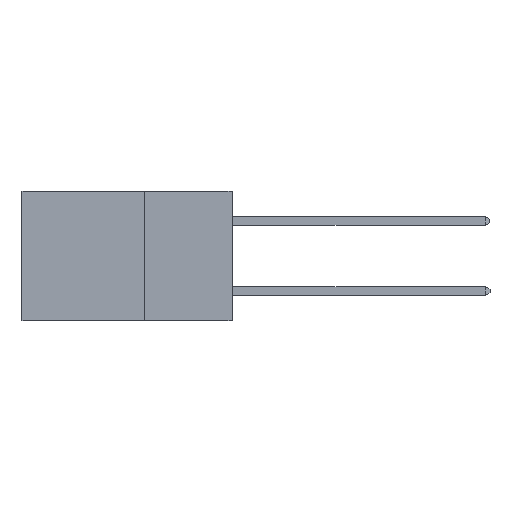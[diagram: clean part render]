
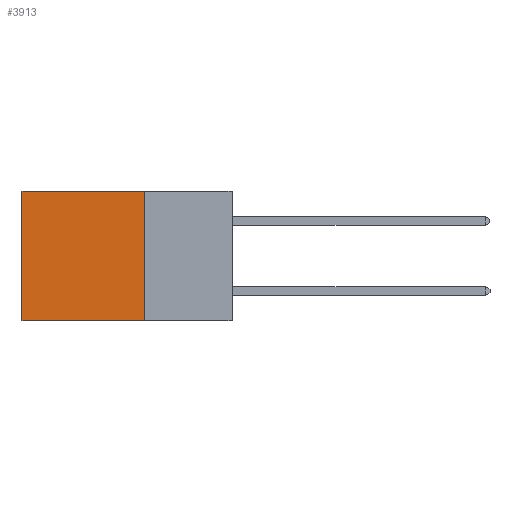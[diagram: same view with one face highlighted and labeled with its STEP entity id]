
A CAD part, left-side view. The second image highlights one B-rep face of the part: STEP entity #3913.
In plain terms, the highlighted planar face has unit normal (-1, 0, 0).
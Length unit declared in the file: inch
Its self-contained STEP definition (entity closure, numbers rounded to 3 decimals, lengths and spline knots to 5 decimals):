
#161 = VERTEX_POINT ( 'NONE', #17658 ) ;
#2437 = EDGE_CURVE ( 'NONE', #161, #13898, #17743, .T. ) ;
#3913 = ADVANCED_FACE ( 'NONE', ( #23017 ), #18521, .F. ) ;
#4895 = AXIS2_PLACEMENT_3D ( 'NONE', #5978, #7819, #20319 ) ;
#4899 = DIRECTION ( 'NONE',  ( 0., 0., -1. ) ) ;
#5817 = CARTESIAN_POINT ( 'NONE',  ( 0.2875, 0.25, -0.37 ) ) ;
#5978 = CARTESIAN_POINT ( 'NONE',  ( 0.2875, 0.25, 0. ) ) ;
#6065 = EDGE_LOOP ( 'NONE', ( #21045, #9711, #15027, #20027 ) ) ;
#6072 = EDGE_CURVE ( 'NONE', #22263, #13898, #16284, .T. ) ;
#6254 = CARTESIAN_POINT ( 'NONE',  ( 0.2875, 0.25, 0. ) ) ;
#6277 = EDGE_CURVE ( 'NONE', #7424, #22263, #7571, .T. ) ;
#6336 = DIRECTION ( 'NONE',  ( 0., 0., -1. ) ) ;
#7301 = CARTESIAN_POINT ( 'NONE',  ( 0.2875, 0.25, 0. ) ) ;
#7424 = VERTEX_POINT ( 'NONE', #19966 ) ;
#7571 = LINE ( 'NONE', #7301, #21841 ) ;
#7819 = DIRECTION ( 'NONE',  ( 1., 0., 0. ) ) ;
#8804 = VECTOR ( 'NONE', #11307, 39.37008 ) ;
#9711 = ORIENTED_EDGE ( 'NONE', *, *, #2437, .F. ) ;
#10094 = EDGE_CURVE ( 'NONE', #7424, #161, #15143, .T. ) ;
#11307 = DIRECTION ( 'NONE',  ( 0., 1., 0. ) ) ;
#13898 = VERTEX_POINT ( 'NONE', #19882 ) ;
#14574 = VECTOR ( 'NONE', #6336, 39.37008 ) ;
#15027 = ORIENTED_EDGE ( 'NONE', *, *, #10094, .F. ) ;
#15143 = LINE ( 'NONE', #6254, #14574 ) ;
#15743 = CARTESIAN_POINT ( 'NONE',  ( 0.2875, 0.6, 0. ) ) ;
#16284 = LINE ( 'NONE', #15743, #21576 ) ;
#17658 = CARTESIAN_POINT ( 'NONE',  ( 0.2875, 0.25, -0.37 ) ) ;
#17743 = LINE ( 'NONE', #5817, #8804 ) ;
#18521 = PLANE ( 'NONE',  #4895 ) ;
#19834 = DIRECTION ( 'NONE',  ( 0., 1., 0. ) ) ;
#19882 = CARTESIAN_POINT ( 'NONE',  ( 0.2875, 0.6, -0.37 ) ) ;
#19966 = CARTESIAN_POINT ( 'NONE',  ( 0.2875, 0.25, 0. ) ) ;
#20027 = ORIENTED_EDGE ( 'NONE', *, *, #6277, .T. ) ;
#20319 = DIRECTION ( 'NONE',  ( 0., 0., -1. ) ) ;
#21045 = ORIENTED_EDGE ( 'NONE', *, *, #6072, .T. ) ;
#21576 = VECTOR ( 'NONE', #4899, 39.37008 ) ;
#21841 = VECTOR ( 'NONE', #19834, 39.37008 ) ;
#22263 = VERTEX_POINT ( 'NONE', #22946 ) ;
#22946 = CARTESIAN_POINT ( 'NONE',  ( 0.2875, 0.6, 0. ) ) ;
#23017 = FACE_OUTER_BOUND ( 'NONE', #6065, .T. ) ;
